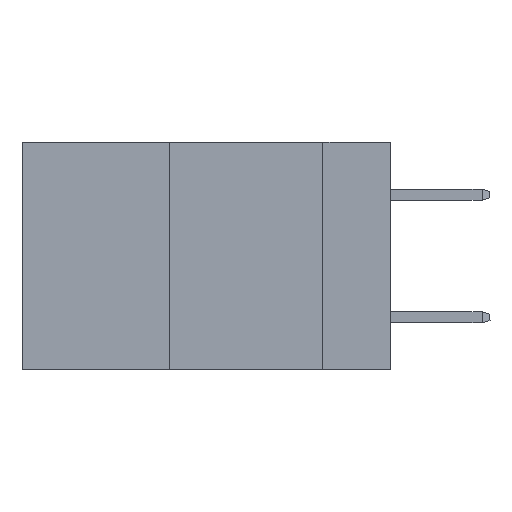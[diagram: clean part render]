
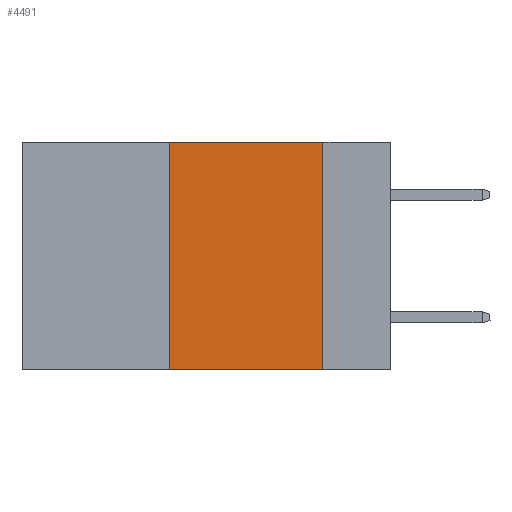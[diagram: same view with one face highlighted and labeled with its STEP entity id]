
A CAD part, left-side view. The second image highlights one B-rep face of the part: STEP entity #4491.
In plain terms, the highlighted planar face has unit normal (-1, 0, 0).
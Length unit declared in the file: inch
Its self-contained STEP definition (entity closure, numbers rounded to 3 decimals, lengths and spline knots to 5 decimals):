
#349 = CARTESIAN_POINT ( 'NONE',  ( 0., 0.11, 0. ) ) ;
#461 = EDGE_CURVE ( 'NONE', #16135, #15453, #5442, .T. ) ;
#609 = CARTESIAN_POINT ( 'NONE',  ( 0., 0.36, 0. ) ) ;
#1128 = VERTEX_POINT ( 'NONE', #7636 ) ;
#1676 = VECTOR ( 'NONE', #14853, 39.37008 ) ;
#3542 = LINE ( 'NONE', #5350, #10857 ) ;
#3792 = CARTESIAN_POINT ( 'NONE',  ( 0., 0.36, 0. ) ) ;
#3862 = VERTEX_POINT ( 'NONE', #609 ) ;
#4491 = ADVANCED_FACE ( 'NONE', ( #13359 ), #10841, .F. ) ;
#5302 = EDGE_CURVE ( 'NONE', #3862, #1128, #3542, .T. ) ;
#5350 = CARTESIAN_POINT ( 'NONE',  ( 0., 0.6, 0. ) ) ;
#5415 = ORIENTED_EDGE ( 'NONE', *, *, #17106, .F. ) ;
#5442 = LINE ( 'NONE', #15590, #5878 ) ;
#5878 = VECTOR ( 'NONE', #11596, 39.37008 ) ;
#7636 = CARTESIAN_POINT ( 'NONE',  ( 0., 0.11, 0. ) ) ;
#7863 = EDGE_CURVE ( 'NONE', #1128, #15453, #16568, .T. ) ;
#8868 = ORIENTED_EDGE ( 'NONE', *, *, #7863, .F. ) ;
#9314 = ORIENTED_EDGE ( 'NONE', *, *, #461, .T. ) ;
#9405 = DIRECTION ( 'NONE',  ( 0., 0., -1. ) ) ;
#10718 = VECTOR ( 'NONE', #18208, 39.37008 ) ;
#10841 = PLANE ( 'NONE',  #18628 ) ;
#10857 = VECTOR ( 'NONE', #12635, 39.37008 ) ;
#11596 = DIRECTION ( 'NONE',  ( 0., -1., 0. ) ) ;
#12635 = DIRECTION ( 'NONE',  ( 0., -1., 0. ) ) ;
#13311 = CARTESIAN_POINT ( 'NONE',  ( 0., 0.36, -0.37 ) ) ;
#13359 = FACE_OUTER_BOUND ( 'NONE', #13419, .T. ) ;
#13419 = EDGE_LOOP ( 'NONE', ( #8868, #16495, #5415, #9314 ) ) ;
#14513 = LINE ( 'NONE', #3792, #10718 ) ;
#14853 = DIRECTION ( 'NONE',  ( 0., 0., -1. ) ) ;
#15111 = CARTESIAN_POINT ( 'NONE',  ( 0., 0.11, -0.37 ) ) ;
#15130 = CARTESIAN_POINT ( 'NONE',  ( 0., 0.6, 0. ) ) ;
#15453 = VERTEX_POINT ( 'NONE', #15111 ) ;
#15590 = CARTESIAN_POINT ( 'NONE',  ( 0., 0.6, -0.37 ) ) ;
#16135 = VERTEX_POINT ( 'NONE', #13311 ) ;
#16495 = ORIENTED_EDGE ( 'NONE', *, *, #5302, .F. ) ;
#16568 = LINE ( 'NONE', #349, #1676 ) ;
#17106 = EDGE_CURVE ( 'NONE', #16135, #3862, #14513, .T. ) ;
#17975 = DIRECTION ( 'NONE',  ( 1., 0., 0. ) ) ;
#18208 = DIRECTION ( 'NONE',  ( 0., 0., 1. ) ) ;
#18628 = AXIS2_PLACEMENT_3D ( 'NONE', #15130, #17975, #9405 ) ;
